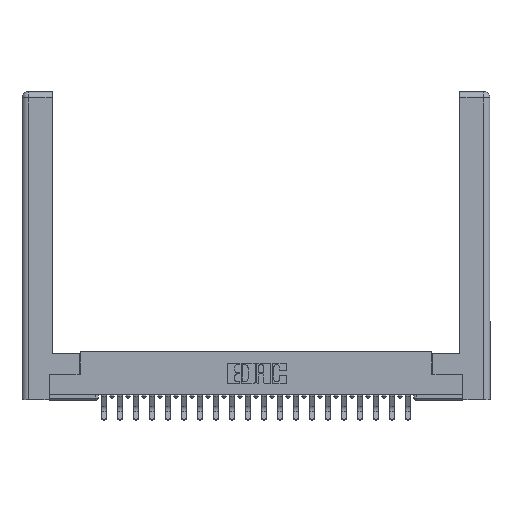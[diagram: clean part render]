
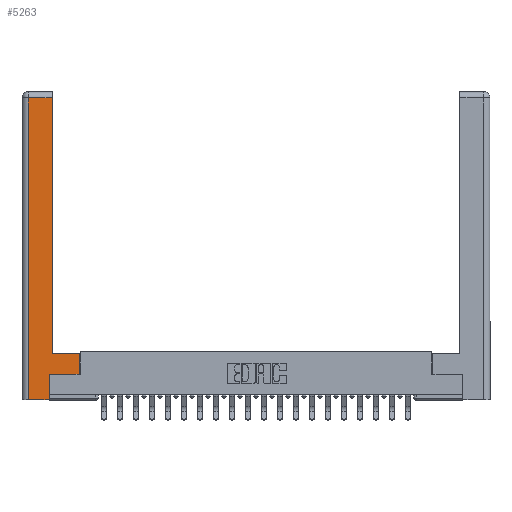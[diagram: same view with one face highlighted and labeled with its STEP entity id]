
A CAD part, top view. The second image highlights one B-rep face of the part: STEP entity #5263.
In plain terms, the highlighted planar face has unit normal (0, 0, 1).
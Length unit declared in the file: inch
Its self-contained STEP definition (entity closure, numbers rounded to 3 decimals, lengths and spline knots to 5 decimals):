
#124 = DIRECTION ( 'NONE',  ( 0., 1., 0. ) ) ;
#279 = CARTESIAN_POINT ( 'NONE',  ( 0.0615, 2.94, 0. ) ) ;
#447 = PLANE ( 'NONE',  #2411 ) ;
#1115 = CARTESIAN_POINT ( 'NONE',  ( 0., 0., 0. ) ) ;
#1710 = VECTOR ( 'NONE', #11175, 39.37008 ) ;
#1841 = ORIENTED_EDGE ( 'NONE', *, *, #9451, .T. ) ;
#2165 = CARTESIAN_POINT ( 'NONE',  ( 0.265, 0., 0. ) ) ;
#2411 = AXIS2_PLACEMENT_3D ( 'NONE', #1115, #12008, #3063 ) ;
#2580 = LINE ( 'NONE', #3156, #12111 ) ;
#2705 = EDGE_CURVE ( 'NONE', #21189, #13352, #12337, .T. ) ;
#2935 = EDGE_CURVE ( 'NONE', #13352, #7824, #11203, .T. ) ;
#3063 = DIRECTION ( 'NONE',  ( -1., 0., 0. ) ) ;
#3117 = CARTESIAN_POINT ( 'NONE',  ( 0.295, 3., 0. ) ) ;
#3156 = CARTESIAN_POINT ( 'NONE',  ( 0.565, 0.45, 0. ) ) ;
#3410 = VECTOR ( 'NONE', #6433, 39.37008 ) ;
#3821 = ORIENTED_EDGE ( 'NONE', *, *, #22287, .T. ) ;
#3846 = CARTESIAN_POINT ( 'NONE',  ( 0.265, 0., 0. ) ) ;
#3916 = CARTESIAN_POINT ( 'NONE',  ( 0.565, 0.245, 0. ) ) ;
#4351 = VERTEX_POINT ( 'NONE', #10758 ) ;
#5087 = CARTESIAN_POINT ( 'NONE',  ( 0.295, 0.45, 0. ) ) ;
#5263 = ADVANCED_FACE ( 'NONE', ( #22627 ), #447, .F. ) ;
#5807 = DIRECTION ( 'NONE',  ( 1., 0., 0. ) ) ;
#6433 = DIRECTION ( 'NONE',  ( 0., -1., 0. ) ) ;
#7267 = LINE ( 'NONE', #5087, #15644 ) ;
#7824 = VERTEX_POINT ( 'NONE', #14889 ) ;
#8193 = LINE ( 'NONE', #17055, #3410 ) ;
#8359 = DIRECTION ( 'NONE',  ( 0., 1., 0. ) ) ;
#9298 = ORIENTED_EDGE ( 'NONE', *, *, #22943, .T. ) ;
#9451 = EDGE_CURVE ( 'NONE', #17841, #20847, #15705, .T. ) ;
#10013 = ORIENTED_EDGE ( 'NONE', *, *, #2935, .T. ) ;
#10079 = VECTOR ( 'NONE', #19832, 39.37008 ) ;
#10484 = ORIENTED_EDGE ( 'NONE', *, *, #21297, .T. ) ;
#10586 = ORIENTED_EDGE ( 'NONE', *, *, #21795, .T. ) ;
#10646 = EDGE_CURVE ( 'NONE', #4351, #21189, #7267, .T. ) ;
#10758 = CARTESIAN_POINT ( 'NONE',  ( 0.565, 0.45, 0. ) ) ;
#11175 = DIRECTION ( 'NONE',  ( 1., 0., 0. ) ) ;
#11203 = LINE ( 'NONE', #279, #10079 ) ;
#12008 = DIRECTION ( 'NONE',  ( 0., 0., -1. ) ) ;
#12111 = VECTOR ( 'NONE', #8359, 39.37008 ) ;
#12337 = LINE ( 'NONE', #3117, #20731 ) ;
#12974 = EDGE_LOOP ( 'NONE', ( #18453, #10013, #10586, #9298, #1841, #3821, #10484, #13409 ) ) ;
#13341 = CARTESIAN_POINT ( 'NONE',  ( 0.295, 0.45, 0. ) ) ;
#13352 = VERTEX_POINT ( 'NONE', #21180 ) ;
#13409 = ORIENTED_EDGE ( 'NONE', *, *, #10646, .T. ) ;
#13760 = VECTOR ( 'NONE', #124, 39.37008 ) ;
#13995 = DIRECTION ( 'NONE',  ( 0., 1., 0. ) ) ;
#14243 = DIRECTION ( 'NONE',  ( -1., 0., 0. ) ) ;
#14630 = CARTESIAN_POINT ( 'NONE',  ( 0.565, 0.245, 0. ) ) ;
#14889 = CARTESIAN_POINT ( 'NONE',  ( 0.0615, 2.94, 0. ) ) ;
#15513 = VERTEX_POINT ( 'NONE', #14630 ) ;
#15644 = VECTOR ( 'NONE', #14243, 39.37008 ) ;
#15705 = LINE ( 'NONE', #21459, #13760 ) ;
#16662 = VERTEX_POINT ( 'NONE', #19666 ) ;
#16851 = VECTOR ( 'NONE', #5807, 39.37008 ) ;
#17055 = CARTESIAN_POINT ( 'NONE',  ( 0.0615, 0., 0. ) ) ;
#17841 = VERTEX_POINT ( 'NONE', #3846 ) ;
#18453 = ORIENTED_EDGE ( 'NONE', *, *, #2705, .T. ) ;
#19666 = CARTESIAN_POINT ( 'NONE',  ( 0.0615, 0., 0. ) ) ;
#19832 = DIRECTION ( 'NONE',  ( -1., 0., 0. ) ) ;
#20731 = VECTOR ( 'NONE', #13995, 39.37008 ) ;
#20847 = VERTEX_POINT ( 'NONE', #21678 ) ;
#21180 = CARTESIAN_POINT ( 'NONE',  ( 0.295, 2.94, 0. ) ) ;
#21189 = VERTEX_POINT ( 'NONE', #13341 ) ;
#21297 = EDGE_CURVE ( 'NONE', #15513, #4351, #2580, .T. ) ;
#21378 = LINE ( 'NONE', #3916, #16851 ) ;
#21459 = CARTESIAN_POINT ( 'NONE',  ( 0.265, 0.245, 0. ) ) ;
#21678 = CARTESIAN_POINT ( 'NONE',  ( 0.265, 0.245, 0. ) ) ;
#21795 = EDGE_CURVE ( 'NONE', #7824, #16662, #8193, .T. ) ;
#22287 = EDGE_CURVE ( 'NONE', #20847, #15513, #21378, .T. ) ;
#22467 = LINE ( 'NONE', #2165, #1710 ) ;
#22627 = FACE_OUTER_BOUND ( 'NONE', #12974, .T. ) ;
#22943 = EDGE_CURVE ( 'NONE', #16662, #17841, #22467, .T. ) ;
